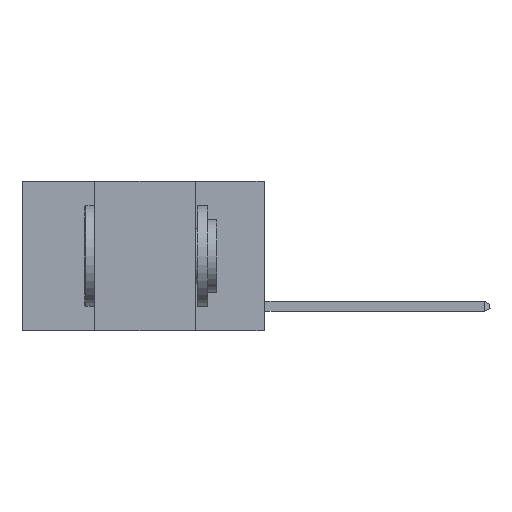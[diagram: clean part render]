
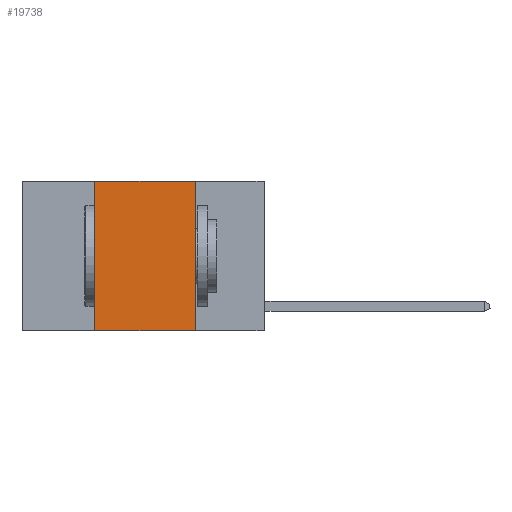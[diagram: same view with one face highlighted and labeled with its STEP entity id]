
A CAD part, left-side view. The second image highlights one B-rep face of the part: STEP entity #19738.
In plain terms, the highlighted planar face has unit normal (-1, 0, 0).
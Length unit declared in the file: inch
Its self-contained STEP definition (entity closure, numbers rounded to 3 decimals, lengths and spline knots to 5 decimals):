
#93 = EDGE_CURVE ( 'NONE', #18716, #3038, #11864, .T. ) ;
#1786 = EDGE_CURVE ( 'NONE', #11481, #3038, #2448, .T. ) ;
#2448 = LINE ( 'NONE', #14096, #19874 ) ;
#3038 = VERTEX_POINT ( 'NONE', #21853 ) ;
#3486 = CARTESIAN_POINT ( 'NONE',  ( 0., 0.6, 0. ) ) ;
#4209 = VERTEX_POINT ( 'NONE', #13228 ) ;
#4480 = ORIENTED_EDGE ( 'NONE', *, *, #9695, .F. ) ;
#5108 = CARTESIAN_POINT ( 'NONE',  ( 0., 0.42, -0.37 ) ) ;
#5407 = ORIENTED_EDGE ( 'NONE', *, *, #1786, .F. ) ;
#5579 = DIRECTION ( 'NONE',  ( 0., 0., -1. ) ) ;
#7419 = FACE_OUTER_BOUND ( 'NONE', #18536, .T. ) ;
#7808 = CARTESIAN_POINT ( 'NONE',  ( 0., 0.6, -0.37 ) ) ;
#9695 = EDGE_CURVE ( 'NONE', #4209, #11481, #25161, .T. ) ;
#10969 = VECTOR ( 'NONE', #21414, 39.37008 ) ;
#11481 = VERTEX_POINT ( 'NONE', #12041 ) ;
#11864 = LINE ( 'NONE', #7808, #10969 ) ;
#12041 = CARTESIAN_POINT ( 'NONE',  ( 0., 0.17, 0. ) ) ;
#13228 = CARTESIAN_POINT ( 'NONE',  ( 0., 0.42, 0. ) ) ;
#14096 = CARTESIAN_POINT ( 'NONE',  ( 0., 0.17, 0. ) ) ;
#14579 = AXIS2_PLACEMENT_3D ( 'NONE', #3486, #21284, #5579 ) ;
#14947 = VECTOR ( 'NONE', #25581, 39.37008 ) ;
#14967 = CARTESIAN_POINT ( 'NONE',  ( 0., 0.6, 0. ) ) ;
#15945 = ORIENTED_EDGE ( 'NONE', *, *, #18445, .F. ) ;
#17362 = ORIENTED_EDGE ( 'NONE', *, *, #93, .T. ) ;
#17379 = PLANE ( 'NONE',  #14579 ) ;
#18445 = EDGE_CURVE ( 'NONE', #18716, #4209, #25456, .T. ) ;
#18536 = EDGE_LOOP ( 'NONE', ( #5407, #4480, #15945, #17362 ) ) ;
#18716 = VERTEX_POINT ( 'NONE', #5108 ) ;
#19738 = ADVANCED_FACE ( 'NONE', ( #7419 ), #17379, .F. ) ;
#19847 = DIRECTION ( 'NONE',  ( 0., 0., -1. ) ) ;
#19874 = VECTOR ( 'NONE', #19847, 39.37008 ) ;
#21284 = DIRECTION ( 'NONE',  ( 1., 0., 0. ) ) ;
#21368 = DIRECTION ( 'NONE',  ( 0., -1., 0. ) ) ;
#21414 = DIRECTION ( 'NONE',  ( 0., -1., 0. ) ) ;
#21853 = CARTESIAN_POINT ( 'NONE',  ( 0., 0.17, -0.37 ) ) ;
#24758 = VECTOR ( 'NONE', #21368, 39.37008 ) ;
#25161 = LINE ( 'NONE', #14967, #24758 ) ;
#25456 = LINE ( 'NONE', #25709, #14947 ) ;
#25581 = DIRECTION ( 'NONE',  ( 0., 0., 1. ) ) ;
#25709 = CARTESIAN_POINT ( 'NONE',  ( 0., 0.42, 0. ) ) ;
